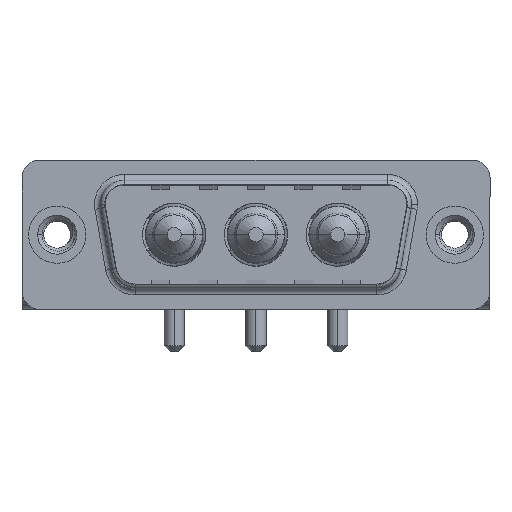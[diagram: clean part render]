
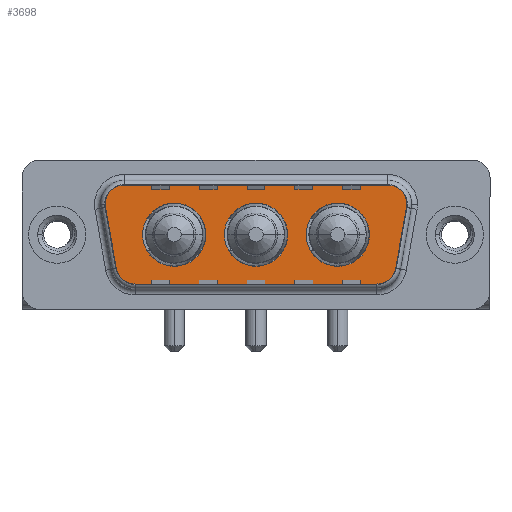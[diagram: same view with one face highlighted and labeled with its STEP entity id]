
A CAD part, top view. The second image highlights one B-rep face of the part: STEP entity #3698.
In plain terms, the highlighted planar face has unit normal (0, 0, 1).
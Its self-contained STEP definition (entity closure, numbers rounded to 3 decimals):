
#39 = ORIENTED_EDGE ( 'NONE', *, *, #12974, .F. ) ;
#79 = AXIS2_PLACEMENT_3D ( 'NONE', #8349, #12549, #2985 ) ;
#268 = EDGE_CURVE ( 'NONE', #856, #5265, #292, .T. ) ;
#284 = EDGE_CURVE ( 'NONE', #4210, #10667, #2003, .T. ) ;
#292 = CIRCLE ( 'NONE', #79, 2. ) ;
#321 = EDGE_CURVE ( 'NONE', #8921, #8231, #12628, .T. ) ;
#377 = CARTESIAN_POINT ( 'NONE',  ( 6.434, -4.9, 0. ) ) ;
#402 = VECTOR ( 'NONE', #7628, 1000. ) ;
#474 = DIRECTION ( 'NONE',  ( 1., 0., 0. ) ) ;
#536 = CARTESIAN_POINT ( 'NONE',  ( 26.866, -2.9, 0. ) ) ;
#670 = FACE_OUTER_BOUND ( 'NONE', #7726, .T. ) ;
#853 = DIRECTION ( 'NONE',  ( -1., 0., 0. ) ) ;
#856 = VERTEX_POINT ( 'NONE', #8681 ) ;
#897 = DIRECTION ( 'NONE',  ( 0., 0., 1. ) ) ;
#1040 = CARTESIAN_POINT ( 'NONE',  ( 16.65, 0., 0. ) ) ;
#1065 = AXIS2_PLACEMENT_3D ( 'NONE', #11605, #7293, #5168 ) ;
#1381 = AXIS2_PLACEMENT_3D ( 'NONE', #10539, #3221, #9556 ) ;
#1486 = CARTESIAN_POINT ( 'NONE',  ( 19.3, 0., 0. ) ) ;
#1515 = VERTEX_POINT ( 'NONE', #11976 ) ;
#1599 = CARTESIAN_POINT ( 'NONE',  ( 29.889, 2.9, 0. ) ) ;
#1682 = CARTESIAN_POINT ( 'NONE',  ( 23.5, 0., 0. ) ) ;
#1717 = CIRCLE ( 'NONE', #1065, 2. ) ;
#1775 = EDGE_CURVE ( 'NONE', #12428, #5484, #5134, .T. ) ;
#2003 = LINE ( 'NONE', #10578, #12405 ) ;
#2519 = CARTESIAN_POINT ( 'NONE',  ( 27.889, 2.9, 0. ) ) ;
#2554 = VERTEX_POINT ( 'NONE', #377 ) ;
#2805 = ORIENTED_EDGE ( 'NONE', *, *, #12213, .F. ) ;
#2849 = LINE ( 'NONE', #8142, #7178 ) ;
#2871 = CARTESIAN_POINT ( 'NONE',  ( 6.434, -4.9, 0. ) ) ;
#2907 = EDGE_CURVE ( 'NONE', #3227, #4210, #6917, .T. ) ;
#2926 = EDGE_CURVE ( 'NONE', #8231, #8921, #10240, .T. ) ;
#2983 = CARTESIAN_POINT ( 'NONE',  ( 5.411, 4.9, 0. ) ) ;
#2985 = DIRECTION ( 'NONE',  ( 1., 0., 0. ) ) ;
#3041 = CARTESIAN_POINT ( 'NONE',  ( 12.45, 0., 0. ) ) ;
#3221 = DIRECTION ( 'NONE',  ( 0., 0., 1. ) ) ;
#3227 = VERTEX_POINT ( 'NONE', #1599 ) ;
#3329 = CIRCLE ( 'NONE', #13002, 2. ) ;
#3564 = DIRECTION ( 'NONE',  ( -1., 0., 0. ) ) ;
#3637 = AXIS2_PLACEMENT_3D ( 'NONE', #13623, #5127, #853 ) ;
#3698 = ADVANCED_FACE ( 'NONE', ( #6591, #10826, #5564, #670 ), #11237, .T. ) ;
#3816 = CARTESIAN_POINT ( 'NONE',  ( 27.889, 4.9, 0. ) ) ;
#3833 = AXIS2_PLACEMENT_3D ( 'NONE', #1040, #897, #11538 ) ;
#3846 = DIRECTION ( 'NONE',  ( 1., 0., 0. ) ) ;
#4115 = AXIS2_PLACEMENT_3D ( 'NONE', #2519, #4650, #3564 ) ;
#4210 = VERTEX_POINT ( 'NONE', #3816 ) ;
#4299 = CARTESIAN_POINT ( 'NONE',  ( 14., 0., 0. ) ) ;
#4486 = DIRECTION ( 'NONE',  ( 1., 0., 0. ) ) ;
#4650 = DIRECTION ( 'NONE',  ( 0., 0., 1. ) ) ;
#4864 = VERTEX_POINT ( 'NONE', #3041 ) ;
#4950 = EDGE_CURVE ( 'NONE', #1515, #3227, #12257, .T. ) ;
#5034 = EDGE_LOOP ( 'NONE', ( #5184, #10514 ) ) ;
#5127 = DIRECTION ( 'NONE',  ( 0., 0., 1. ) ) ;
#5134 = CIRCLE ( 'NONE', #6478, 2.65 ) ;
#5168 = DIRECTION ( 'NONE',  ( 1., 0., 0. ) ) ;
#5184 = ORIENTED_EDGE ( 'NONE', *, *, #2926, .F. ) ;
#5265 = VERTEX_POINT ( 'NONE', #6293 ) ;
#5484 = VERTEX_POINT ( 'NONE', #9891 ) ;
#5564 = FACE_BOUND ( 'NONE', #13346, .T. ) ;
#5634 = CARTESIAN_POINT ( 'NONE',  ( 29.859, 2.553, 0. ) ) ;
#5644 = ORIENTED_EDGE ( 'NONE', *, *, #2907, .T. ) ;
#5649 = EDGE_CURVE ( 'NONE', #12301, #12662, #2849, .T. ) ;
#5715 = CARTESIAN_POINT ( 'NONE',  ( 7.15, 0., 0. ) ) ;
#5786 = DIRECTION ( 'NONE',  ( -1., 0., 0. ) ) ;
#5852 = EDGE_CURVE ( 'NONE', #4864, #10600, #12275, .T. ) ;
#6293 = CARTESIAN_POINT ( 'NONE',  ( 28.836, -3.247, 0. ) ) ;
#6318 = AXIS2_PLACEMENT_3D ( 'NONE', #6677, #12967, #4486 ) ;
#6478 = AXIS2_PLACEMENT_3D ( 'NONE', #9935, #7705, #474 ) ;
#6591 = FACE_BOUND ( 'NONE', #5034, .T. ) ;
#6677 = CARTESIAN_POINT ( 'NONE',  ( 9.8, 0., 0. ) ) ;
#6767 = EDGE_CURVE ( 'NONE', #10667, #12301, #1717, .T. ) ;
#6842 = EDGE_CURVE ( 'NONE', #5265, #1515, #7436, .T. ) ;
#6917 = CIRCLE ( 'NONE', #3637, 2. ) ;
#7178 = VECTOR ( 'NONE', #11138, 1000. ) ;
#7256 = CARTESIAN_POINT ( 'NONE',  ( 16.65, 0., 0. ) ) ;
#7293 = DIRECTION ( 'NONE',  ( 0., 0., 1. ) ) ;
#7406 = CARTESIAN_POINT ( 'NONE',  ( 4.464, -3.247, 0. ) ) ;
#7436 = LINE ( 'NONE', #5634, #402 ) ;
#7628 = DIRECTION ( 'NONE',  ( 0.174, 0.985, 0. ) ) ;
#7629 = ORIENTED_EDGE ( 'NONE', *, *, #9136, .T. ) ;
#7705 = DIRECTION ( 'NONE',  ( 0., 0., 1. ) ) ;
#7726 = EDGE_LOOP ( 'NONE', ( #8517, #11938, #10860, #5644, #10441, #9919, #13451, #7629, #11649 ) ) ;
#8142 = CARTESIAN_POINT ( 'NONE',  ( 3.441, 2.553, 0. ) ) ;
#8231 = VERTEX_POINT ( 'NONE', #1486 ) ;
#8349 = CARTESIAN_POINT ( 'NONE',  ( 26.866, -2.9, 0. ) ) ;
#8406 = ORIENTED_EDGE ( 'NONE', *, *, #1775, .F. ) ;
#8517 = ORIENTED_EDGE ( 'NONE', *, *, #268, .T. ) ;
#8681 = CARTESIAN_POINT ( 'NONE',  ( 26.866, -4.9, 0. ) ) ;
#8921 = VERTEX_POINT ( 'NONE', #4299 ) ;
#8952 = DIRECTION ( 'NONE',  ( 1., 0., 0. ) ) ;
#8973 = CARTESIAN_POINT ( 'NONE',  ( 6.434, -2.9, 0. ) ) ;
#8993 = DIRECTION ( 'NONE',  ( 1., 0., 0. ) ) ;
#9072 = LINE ( 'NONE', #2871, #11495 ) ;
#9136 = EDGE_CURVE ( 'NONE', #12662, #2554, #3329, .T. ) ;
#9218 = DIRECTION ( 'NONE',  ( 0., 0., 1. ) ) ;
#9263 = DIRECTION ( 'NONE',  ( 1., 0., 0. ) ) ;
#9362 = CIRCLE ( 'NONE', #9807, 2.65 ) ;
#9556 = DIRECTION ( 'NONE',  ( 1., 0., 0. ) ) ;
#9595 = EDGE_CURVE ( 'NONE', #2554, #856, #9072, .T. ) ;
#9807 = AXIS2_PLACEMENT_3D ( 'NONE', #1682, #12304, #8993 ) ;
#9891 = CARTESIAN_POINT ( 'NONE',  ( 20.85, 0., 0. ) ) ;
#9919 = ORIENTED_EDGE ( 'NONE', *, *, #6767, .T. ) ;
#9935 = CARTESIAN_POINT ( 'NONE',  ( 23.5, 0., 0. ) ) ;
#10240 = CIRCLE ( 'NONE', #10911, 2.65 ) ;
#10441 = ORIENTED_EDGE ( 'NONE', *, *, #284, .T. ) ;
#10486 = AXIS2_PLACEMENT_3D ( 'NONE', #536, #9218, #8952 ) ;
#10514 = ORIENTED_EDGE ( 'NONE', *, *, #321, .F. ) ;
#10539 = CARTESIAN_POINT ( 'NONE',  ( 9.8, 0., 0. ) ) ;
#10578 = CARTESIAN_POINT ( 'NONE',  ( 5.411, 4.9, 0. ) ) ;
#10599 = EDGE_LOOP ( 'NONE', ( #8406, #39 ) ) ;
#10600 = VERTEX_POINT ( 'NONE', #5715 ) ;
#10628 = ORIENTED_EDGE ( 'NONE', *, *, #5852, .F. ) ;
#10667 = VERTEX_POINT ( 'NONE', #2983 ) ;
#10826 = FACE_BOUND ( 'NONE', #10599, .T. ) ;
#10860 = ORIENTED_EDGE ( 'NONE', *, *, #4950, .T. ) ;
#10911 = AXIS2_PLACEMENT_3D ( 'NONE', #7256, #11351, #9263 ) ;
#10938 = CARTESIAN_POINT ( 'NONE',  ( 3.441, 2.553, 0. ) ) ;
#11087 = CIRCLE ( 'NONE', #1381, 2.65 ) ;
#11138 = DIRECTION ( 'NONE',  ( 0.174, -0.985, 0. ) ) ;
#11237 = PLANE ( 'NONE',  #10486 ) ;
#11309 = DIRECTION ( 'NONE',  ( 0., 0., 1. ) ) ;
#11351 = DIRECTION ( 'NONE',  ( 0., 0., 1. ) ) ;
#11495 = VECTOR ( 'NONE', #3846, 1000. ) ;
#11538 = DIRECTION ( 'NONE',  ( 1., 0., 0. ) ) ;
#11605 = CARTESIAN_POINT ( 'NONE',  ( 5.411, 2.9, 0. ) ) ;
#11649 = ORIENTED_EDGE ( 'NONE', *, *, #9595, .T. ) ;
#11938 = ORIENTED_EDGE ( 'NONE', *, *, #6842, .T. ) ;
#11976 = CARTESIAN_POINT ( 'NONE',  ( 29.859, 2.553, 0. ) ) ;
#12213 = EDGE_CURVE ( 'NONE', #10600, #4864, #11087, .T. ) ;
#12257 = CIRCLE ( 'NONE', #4115, 2. ) ;
#12275 = CIRCLE ( 'NONE', #6318, 2.65 ) ;
#12301 = VERTEX_POINT ( 'NONE', #10938 ) ;
#12304 = DIRECTION ( 'NONE',  ( 0., 0., 1. ) ) ;
#12405 = VECTOR ( 'NONE', #13456, 1000. ) ;
#12428 = VERTEX_POINT ( 'NONE', #12919 ) ;
#12549 = DIRECTION ( 'NONE',  ( 0., 0., 1. ) ) ;
#12628 = CIRCLE ( 'NONE', #3833, 2.65 ) ;
#12662 = VERTEX_POINT ( 'NONE', #7406 ) ;
#12919 = CARTESIAN_POINT ( 'NONE',  ( 26.15, 0., 0. ) ) ;
#12967 = DIRECTION ( 'NONE',  ( 0., 0., 1. ) ) ;
#12974 = EDGE_CURVE ( 'NONE', #5484, #12428, #9362, .T. ) ;
#13002 = AXIS2_PLACEMENT_3D ( 'NONE', #8973, #11309, #5786 ) ;
#13346 = EDGE_LOOP ( 'NONE', ( #10628, #2805 ) ) ;
#13451 = ORIENTED_EDGE ( 'NONE', *, *, #5649, .T. ) ;
#13456 = DIRECTION ( 'NONE',  ( -1., 0., 0. ) ) ;
#13623 = CARTESIAN_POINT ( 'NONE',  ( 27.889, 2.9, 0. ) ) ;
